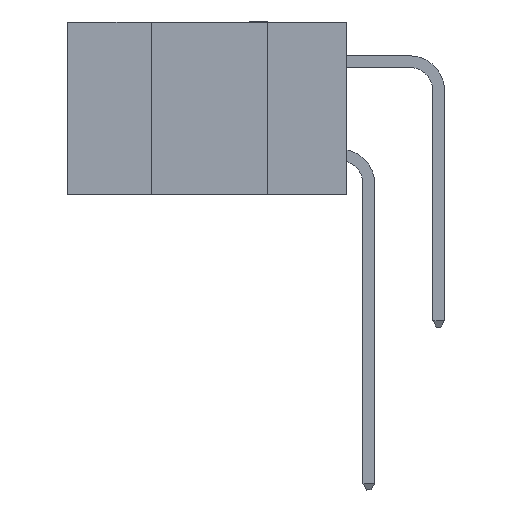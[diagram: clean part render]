
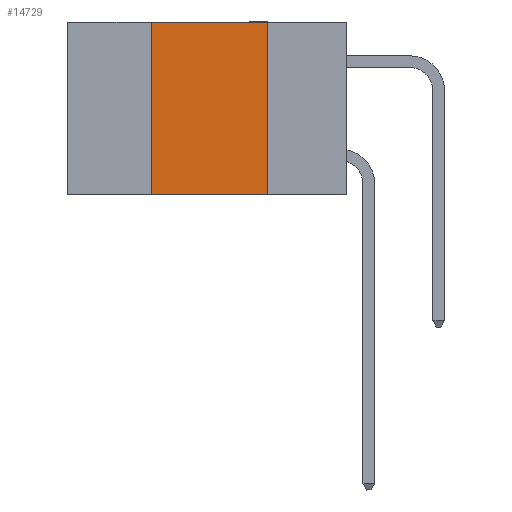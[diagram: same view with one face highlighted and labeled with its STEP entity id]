
A CAD part, left-side view. The second image highlights one B-rep face of the part: STEP entity #14729.
In plain terms, the highlighted planar face has unit normal (-1, 0, 0).
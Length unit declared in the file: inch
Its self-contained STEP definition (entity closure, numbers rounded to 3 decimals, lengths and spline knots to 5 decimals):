
#15 = CARTESIAN_POINT ( 'NONE',  ( 0., 0.6, -0.37 ) ) ;
#525 = ORIENTED_EDGE ( 'NONE', *, *, #8988, .T. ) ;
#921 = VERTEX_POINT ( 'NONE', #19410 ) ;
#1719 = AXIS2_PLACEMENT_3D ( 'NONE', #6552, #13234, #9399 ) ;
#3388 = LINE ( 'NONE', #3707, #5569 ) ;
#3707 = CARTESIAN_POINT ( 'NONE',  ( 0., 0.6, 0. ) ) ;
#4381 = VERTEX_POINT ( 'NONE', #13067 ) ;
#5053 = VECTOR ( 'NONE', #16901, 39.37008 ) ;
#5530 = DIRECTION ( 'NONE',  ( 0., 0., -1. ) ) ;
#5569 = VECTOR ( 'NONE', #10379, 39.37008 ) ;
#5878 = LINE ( 'NONE', #17240, #15272 ) ;
#6552 = CARTESIAN_POINT ( 'NONE',  ( 0., 0.6, 0. ) ) ;
#7640 = VERTEX_POINT ( 'NONE', #17988 ) ;
#8691 = CARTESIAN_POINT ( 'NONE',  ( 0., 0.42, -0.37 ) ) ;
#8940 = DIRECTION ( 'NONE',  ( 0., 0., 1. ) ) ;
#8988 = EDGE_CURVE ( 'NONE', #12949, #921, #10263, .T. ) ;
#9015 = EDGE_CURVE ( 'NONE', #4381, #921, #20383, .T. ) ;
#9399 = DIRECTION ( 'NONE',  ( 0., 0., -1. ) ) ;
#10263 = LINE ( 'NONE', #15, #5053 ) ;
#10379 = DIRECTION ( 'NONE',  ( 0., -1., 0. ) ) ;
#12012 = CARTESIAN_POINT ( 'NONE',  ( 0., 0.17, 0. ) ) ;
#12066 = ORIENTED_EDGE ( 'NONE', *, *, #16285, .F. ) ;
#12949 = VERTEX_POINT ( 'NONE', #8691 ) ;
#13067 = CARTESIAN_POINT ( 'NONE',  ( 0., 0.17, 0. ) ) ;
#13234 = DIRECTION ( 'NONE',  ( 1., 0., 0. ) ) ;
#14729 = ADVANCED_FACE ( 'NONE', ( #21508 ), #16492, .F. ) ;
#15272 = VECTOR ( 'NONE', #8940, 39.37008 ) ;
#16285 = EDGE_CURVE ( 'NONE', #12949, #7640, #5878, .T. ) ;
#16492 = PLANE ( 'NONE',  #1719 ) ;
#16901 = DIRECTION ( 'NONE',  ( 0., -1., 0. ) ) ;
#17240 = CARTESIAN_POINT ( 'NONE',  ( 0., 0.42, 0. ) ) ;
#17988 = CARTESIAN_POINT ( 'NONE',  ( 0., 0.42, 0. ) ) ;
#18839 = ORIENTED_EDGE ( 'NONE', *, *, #20570, .F. ) ;
#19410 = CARTESIAN_POINT ( 'NONE',  ( 0., 0.17, -0.37 ) ) ;
#19898 = ORIENTED_EDGE ( 'NONE', *, *, #9015, .F. ) ;
#20383 = LINE ( 'NONE', #12012, #21437 ) ;
#20570 = EDGE_CURVE ( 'NONE', #7640, #4381, #3388, .T. ) ;
#20962 = EDGE_LOOP ( 'NONE', ( #19898, #18839, #12066, #525 ) ) ;
#21437 = VECTOR ( 'NONE', #5530, 39.37008 ) ;
#21508 = FACE_OUTER_BOUND ( 'NONE', #20962, .T. ) ;
